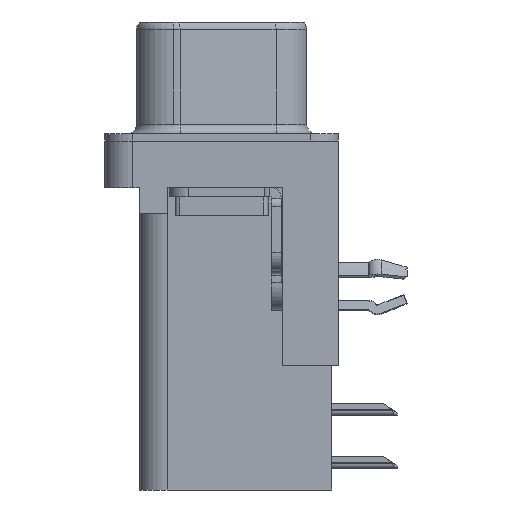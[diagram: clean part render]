
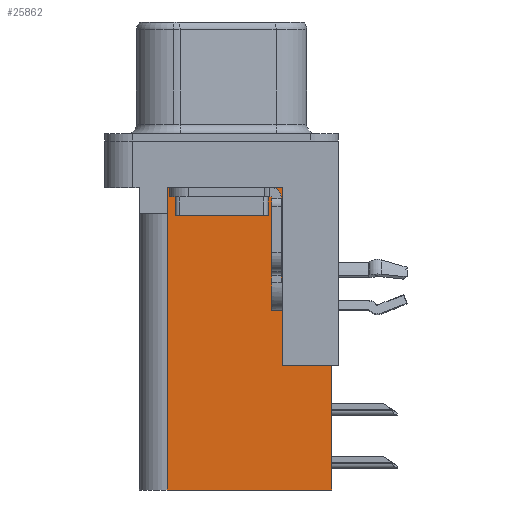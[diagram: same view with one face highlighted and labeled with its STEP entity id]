
A CAD part, left-side view. The second image highlights one B-rep face of the part: STEP entity #25862.
In plain terms, the highlighted planar face has unit normal (-1, 0, 0).
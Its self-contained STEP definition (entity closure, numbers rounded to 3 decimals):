
#167 = VERTEX_POINT ( 'NONE', #8305 ) ;
#943 = CARTESIAN_POINT ( 'NONE',  ( 3.79, -3.295, -2.5 ) ) ;
#1044 = CARTESIAN_POINT ( 'NONE',  ( 3.79, 2.895, -3.9 ) ) ;
#1067 = EDGE_CURVE ( 'NONE', #4889, #26020, #7148, .T. ) ;
#1073 = VERTEX_POINT ( 'NONE', #20123 ) ;
#2081 = VECTOR ( 'NONE', #3425, 1000. ) ;
#2252 = VERTEX_POINT ( 'NONE', #24718 ) ;
#3425 = DIRECTION ( 'NONE',  ( 0., 1., 0. ) ) ;
#4005 = CARTESIAN_POINT ( 'NONE',  ( 3.79, -3.295, -18.76 ) ) ;
#4474 = CARTESIAN_POINT ( 'NONE',  ( 3.79, 0., -3.9 ) ) ;
#4889 = VERTEX_POINT ( 'NONE', #20992 ) ;
#5783 = DIRECTION ( 'NONE',  ( 0., 1., 0. ) ) ;
#6203 = CARTESIAN_POINT ( 'NONE',  ( 3.79, 2.895, -3.9 ) ) ;
#6204 = EDGE_CURVE ( 'NONE', #2252, #4889, #17517, .T. ) ;
#6801 = CARTESIAN_POINT ( 'NONE',  ( 3.79, -5.925, -12.05 ) ) ;
#6894 = EDGE_CURVE ( 'NONE', #8264, #2252, #24528, .T. ) ;
#7057 = VECTOR ( 'NONE', #7518, 1000. ) ;
#7148 = LINE ( 'NONE', #25034, #7057 ) ;
#7380 = EDGE_CURVE ( 'NONE', #8264, #167, #24308, .T. ) ;
#7518 = DIRECTION ( 'NONE',  ( 0., 0., 1. ) ) ;
#7579 = EDGE_CURVE ( 'NONE', #167, #1073, #24166, .T. ) ;
#7698 = CARTESIAN_POINT ( 'NONE',  ( 3.79, -3.295, -18.76 ) ) ;
#7800 = PLANE ( 'NONE',  #25152 ) ;
#8264 = VERTEX_POINT ( 'NONE', #6801 ) ;
#8305 = CARTESIAN_POINT ( 'NONE',  ( 3.79, -3.295, -12.05 ) ) ;
#8710 = EDGE_LOOP ( 'NONE', ( #14321, #15099, #19402, #11547, #11458, #10079, #11236, #16561 ) ) ;
#10079 = ORIENTED_EDGE ( 'NONE', *, *, #6894, .F. ) ;
#10250 = DIRECTION ( 'NONE',  ( 0., 0., -1. ) ) ;
#10314 = CARTESIAN_POINT ( 'NONE',  ( 3.79, -6.295, -12.05 ) ) ;
#10749 = DIRECTION ( 'NONE',  ( 0., 0., 1. ) ) ;
#11236 = ORIENTED_EDGE ( 'NONE', *, *, #7380, .T. ) ;
#11458 = ORIENTED_EDGE ( 'NONE', *, *, #6204, .F. ) ;
#11547 = ORIENTED_EDGE ( 'NONE', *, *, #1067, .F. ) ;
#12311 = CARTESIAN_POINT ( 'NONE',  ( 3.79, 2.925, -3.9 ) ) ;
#13511 = DIRECTION ( 'NONE',  ( 0., 1., 0. ) ) ;
#14098 = VECTOR ( 'NONE', #13511, 1000. ) ;
#14265 = LINE ( 'NONE', #943, #14098 ) ;
#14321 = ORIENTED_EDGE ( 'NONE', *, *, #21569, .T. ) ;
#15099 = ORIENTED_EDGE ( 'NONE', *, *, #25545, .T. ) ;
#15369 = CARTESIAN_POINT ( 'NONE',  ( 3.79, 2.895, -2.5 ) ) ;
#16561 = ORIENTED_EDGE ( 'NONE', *, *, #7579, .T. ) ;
#17476 = FACE_OUTER_BOUND ( 'NONE', #8710, .T. ) ;
#17517 = LINE ( 'NONE', #4005, #2081 ) ;
#17694 = DIRECTION ( 'NONE',  ( 1., 0., 0. ) ) ;
#18591 = DIRECTION ( 'NONE',  ( 0., 1., 0. ) ) ;
#18882 = CARTESIAN_POINT ( 'NONE',  ( 3.79, -5.925, -2. ) ) ;
#19188 = EDGE_CURVE ( 'NONE', #19377, #26020, #21179, .T. ) ;
#19308 = VERTEX_POINT ( 'NONE', #15369 ) ;
#19377 = VERTEX_POINT ( 'NONE', #1044 ) ;
#19402 = ORIENTED_EDGE ( 'NONE', *, *, #19188, .T. ) ;
#20123 = CARTESIAN_POINT ( 'NONE',  ( 3.79, -3.295, -2.5 ) ) ;
#20579 = CARTESIAN_POINT ( 'NONE',  ( 3.79, -3.295, -18.76 ) ) ;
#20848 = VECTOR ( 'NONE', #10250, 1000. ) ;
#20866 = DIRECTION ( 'NONE',  ( 0., 0., -1. ) ) ;
#20992 = CARTESIAN_POINT ( 'NONE',  ( 3.79, 2.925, -18.76 ) ) ;
#21179 = LINE ( 'NONE', #4474, #21221 ) ;
#21221 = VECTOR ( 'NONE', #18591, 1000. ) ;
#21372 = LINE ( 'NONE', #6203, #20848 ) ;
#21569 = EDGE_CURVE ( 'NONE', #1073, #19308, #14265, .T. ) ;
#23498 = VECTOR ( 'NONE', #10749, 1000. ) ;
#24125 = DIRECTION ( 'NONE',  ( 0., 1., 0. ) ) ;
#24166 = LINE ( 'NONE', #20579, #23498 ) ;
#24308 = LINE ( 'NONE', #10314, #24589 ) ;
#24528 = LINE ( 'NONE', #18882, #24860 ) ;
#24589 = VECTOR ( 'NONE', #24125, 1000. ) ;
#24718 = CARTESIAN_POINT ( 'NONE',  ( 3.79, -5.925, -18.76 ) ) ;
#24860 = VECTOR ( 'NONE', #20866, 1000. ) ;
#25034 = CARTESIAN_POINT ( 'NONE',  ( 3.79, 2.925, -18.76 ) ) ;
#25152 = AXIS2_PLACEMENT_3D ( 'NONE', #7698, #17694, #5783 ) ;
#25545 = EDGE_CURVE ( 'NONE', #19308, #19377, #21372, .T. ) ;
#25862 = ADVANCED_FACE ( 'NONE', ( #17476 ), #7800, .F. ) ;
#26020 = VERTEX_POINT ( 'NONE', #12311 ) ;
